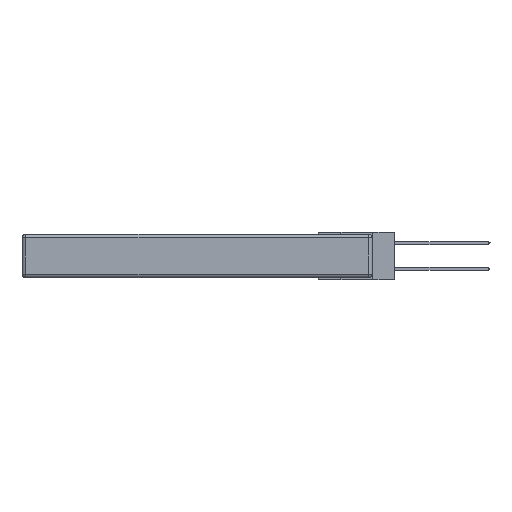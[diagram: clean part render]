
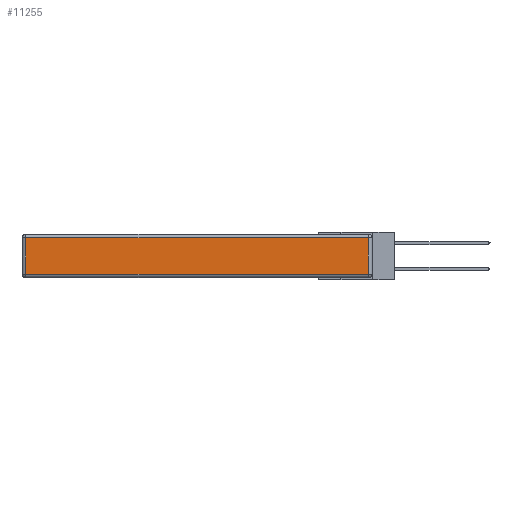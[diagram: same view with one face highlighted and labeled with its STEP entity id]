
A CAD part, left-side view. The second image highlights one B-rep face of the part: STEP entity #11255.
In plain terms, the highlighted planar face has unit normal (-1, 0, 0).
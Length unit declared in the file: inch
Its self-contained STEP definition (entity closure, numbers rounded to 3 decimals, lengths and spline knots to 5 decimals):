
#324 = CARTESIAN_POINT ( 'NONE',  ( 0., 0.03, -0.03 ) ) ;
#482 = DIRECTION ( 'NONE',  ( 0., 0., 1. ) ) ;
#1398 = VERTEX_POINT ( 'NONE', #324 ) ;
#1725 = AXIS2_PLACEMENT_3D ( 'NONE', #9156, #6118, #12093 ) ;
#2236 = CARTESIAN_POINT ( 'NONE',  ( 0., 2.72, -0.313 ) ) ;
#2385 = DIRECTION ( 'NONE',  ( 0., 1., 0. ) ) ;
#2897 = VERTEX_POINT ( 'NONE', #2236 ) ;
#4500 = EDGE_LOOP ( 'NONE', ( #8456, #6968, #17924, #12218 ) ) ;
#4683 = CARTESIAN_POINT ( 'NONE',  ( 0., 2.72, -0.03 ) ) ;
#5543 = VECTOR ( 'NONE', #6607, 39.37008 ) ;
#5769 = LINE ( 'NONE', #12567, #5543 ) ;
#6118 = DIRECTION ( 'NONE',  ( -1., 0., 0. ) ) ;
#6607 = DIRECTION ( 'NONE',  ( 0., 0., -1. ) ) ;
#6758 = VERTEX_POINT ( 'NONE', #4683 ) ;
#6968 = ORIENTED_EDGE ( 'NONE', *, *, #7917, .T. ) ;
#6973 = LINE ( 'NONE', #10629, #18353 ) ;
#7917 = EDGE_CURVE ( 'NONE', #10958, #1398, #15411, .T. ) ;
#8456 = ORIENTED_EDGE ( 'NONE', *, *, #15439, .T. ) ;
#8566 = EDGE_CURVE ( 'NONE', #6758, #2897, #5769, .T. ) ;
#8620 = LINE ( 'NONE', #17170, #10708 ) ;
#9156 = CARTESIAN_POINT ( 'NONE',  ( 0., 0., -0.343 ) ) ;
#10516 = PLANE ( 'NONE',  #1725 ) ;
#10629 = CARTESIAN_POINT ( 'NONE',  ( 0., 0., -0.313 ) ) ;
#10708 = VECTOR ( 'NONE', #2385, 39.37008 ) ;
#10958 = VERTEX_POINT ( 'NONE', #11452 ) ;
#11144 = CARTESIAN_POINT ( 'NONE',  ( 0., 0.03, -0.343 ) ) ;
#11255 = ADVANCED_FACE ( 'NONE', ( #17291 ), #10516, .T. ) ;
#11452 = CARTESIAN_POINT ( 'NONE',  ( 0., 0.03, -0.313 ) ) ;
#11453 = VECTOR ( 'NONE', #482, 39.37008 ) ;
#12093 = DIRECTION ( 'NONE',  ( 0., 0., 1. ) ) ;
#12218 = ORIENTED_EDGE ( 'NONE', *, *, #8566, .T. ) ;
#12567 = CARTESIAN_POINT ( 'NONE',  ( 0., 2.72, -0.343 ) ) ;
#12830 = EDGE_CURVE ( 'NONE', #1398, #6758, #8620, .T. ) ;
#13773 = DIRECTION ( 'NONE',  ( 0., -1., 0. ) ) ;
#15411 = LINE ( 'NONE', #11144, #11453 ) ;
#15439 = EDGE_CURVE ( 'NONE', #2897, #10958, #6973, .T. ) ;
#17170 = CARTESIAN_POINT ( 'NONE',  ( 0., 2.75, -0.03 ) ) ;
#17291 = FACE_OUTER_BOUND ( 'NONE', #4500, .T. ) ;
#17924 = ORIENTED_EDGE ( 'NONE', *, *, #12830, .T. ) ;
#18353 = VECTOR ( 'NONE', #13773, 39.37008 ) ;
